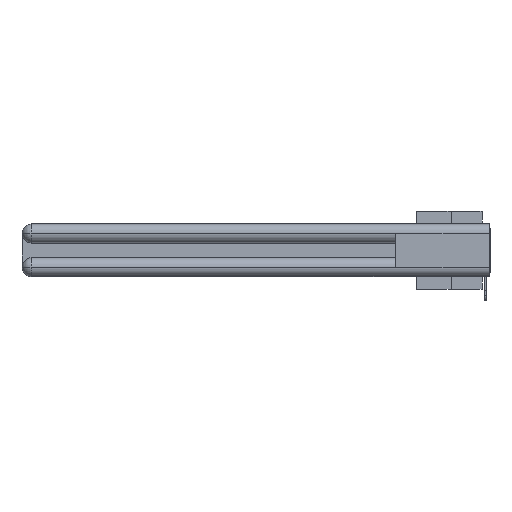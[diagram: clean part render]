
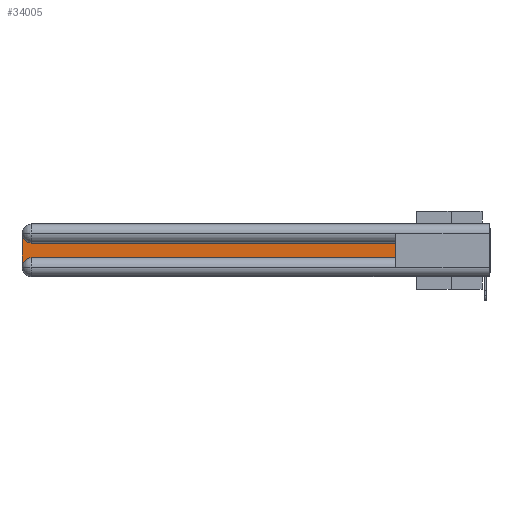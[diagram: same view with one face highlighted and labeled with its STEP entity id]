
A CAD part, left-side view. The second image highlights one B-rep face of the part: STEP entity #34005.
In plain terms, the highlighted planar face has unit normal (-1, 0, 0).
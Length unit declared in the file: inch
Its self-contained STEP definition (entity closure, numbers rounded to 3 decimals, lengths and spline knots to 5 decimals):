
#265 = DIRECTION ( 'NONE',  ( 1., 0., 0. ) ) ;
#384 = CARTESIAN_POINT ( 'NONE',  ( 0.075, 2.94, -0.2775 ) ) ;
#1418 = DIRECTION ( 'NONE',  ( 0., 0., 1. ) ) ;
#1859 = FACE_OUTER_BOUND ( 'NONE', #2344, .T. ) ;
#2344 = EDGE_LOOP ( 'NONE', ( #36586, #9857, #8368, #4734, #7684, #28062 ) ) ;
#3530 = AXIS2_PLACEMENT_3D ( 'NONE', #37875, #265, #41005 ) ;
#4423 = AXIS2_PLACEMENT_3D ( 'NONE', #8294, #18045, #14731 ) ;
#4734 = ORIENTED_EDGE ( 'NONE', *, *, #36474, .T. ) ;
#7265 = DIRECTION ( 'NONE',  ( 1., 0., 0. ) ) ;
#7353 = VERTEX_POINT ( 'NONE', #28153 ) ;
#7684 = ORIENTED_EDGE ( 'NONE', *, *, #11044, .T. ) ;
#8294 = CARTESIAN_POINT ( 'NONE',  ( 0.075, 3., -0.1225 ) ) ;
#8368 = ORIENTED_EDGE ( 'NONE', *, *, #30786, .T. ) ;
#9474 = CARTESIAN_POINT ( 'NONE',  ( 0.075, 3., -0.2175 ) ) ;
#9786 = AXIS2_PLACEMENT_3D ( 'NONE', #384, #7265, #19921 ) ;
#9857 = ORIENTED_EDGE ( 'NONE', *, *, #31177, .T. ) ;
#10422 = LINE ( 'NONE', #29315, #27068 ) ;
#11022 = VERTEX_POINT ( 'NONE', #39094 ) ;
#11044 = EDGE_CURVE ( 'NONE', #16330, #7353, #10422, .T. ) ;
#12972 = DIRECTION ( 'NONE',  ( 0., 0., -1. ) ) ;
#13334 = DIRECTION ( 'NONE',  ( 0., -1., 0. ) ) ;
#14731 = DIRECTION ( 'NONE',  ( 0., 0., -1. ) ) ;
#15416 = CARTESIAN_POINT ( 'NONE',  ( 0.075, 0.6, -0.1225 ) ) ;
#15624 = CARTESIAN_POINT ( 'NONE',  ( 0.075, 2.94, -0.1225 ) ) ;
#16330 = VERTEX_POINT ( 'NONE', #22347 ) ;
#16804 = VECTOR ( 'NONE', #24823, 39.37008 ) ;
#18045 = DIRECTION ( 'NONE',  ( 1., 0., 0. ) ) ;
#19921 = DIRECTION ( 'NONE',  ( 0., 0., -1. ) ) ;
#21067 = VECTOR ( 'NONE', #1418, 39.37008 ) ;
#21129 = CARTESIAN_POINT ( 'NONE',  ( 0.075, 0.6, -0.2175 ) ) ;
#22330 = CARTESIAN_POINT ( 'NONE',  ( 0.075, 0.6, -0.1225 ) ) ;
#22347 = CARTESIAN_POINT ( 'NONE',  ( 0.075, 2.94, -0.2175 ) ) ;
#24222 = LINE ( 'NONE', #21129, #21067 ) ;
#24823 = DIRECTION ( 'NONE',  ( 0., 1., 0. ) ) ;
#27068 = VECTOR ( 'NONE', #13334, 39.37008 ) ;
#27660 = CIRCLE ( 'NONE', #9786, 0.06 ) ;
#28062 = ORIENTED_EDGE ( 'NONE', *, *, #36531, .T. ) ;
#28153 = CARTESIAN_POINT ( 'NONE',  ( 0.075, 0.6, -0.2175 ) ) ;
#28333 = VERTEX_POINT ( 'NONE', #39480 ) ;
#29315 = CARTESIAN_POINT ( 'NONE',  ( 0.075, 0.6, -0.2175 ) ) ;
#29894 = VERTEX_POINT ( 'NONE', #15624 ) ;
#30762 = EDGE_CURVE ( 'NONE', #38937, #29894, #34601, .T. ) ;
#30786 = EDGE_CURVE ( 'NONE', #28333, #11022, #31689, .T. ) ;
#31177 = EDGE_CURVE ( 'NONE', #29894, #28333, #39348, .T. ) ;
#31689 = LINE ( 'NONE', #9474, #32051 ) ;
#32051 = VECTOR ( 'NONE', #12972, 39.37008 ) ;
#34005 = ADVANCED_FACE ( 'NONE', ( #1859 ), #40291, .F. ) ;
#34601 = LINE ( 'NONE', #22330, #16804 ) ;
#36474 = EDGE_CURVE ( 'NONE', #11022, #16330, #27660, .T. ) ;
#36531 = EDGE_CURVE ( 'NONE', #7353, #38937, #24222, .T. ) ;
#36586 = ORIENTED_EDGE ( 'NONE', *, *, #30762, .T. ) ;
#37875 = CARTESIAN_POINT ( 'NONE',  ( 0.075, 2.94, -0.0625 ) ) ;
#38937 = VERTEX_POINT ( 'NONE', #15416 ) ;
#39094 = CARTESIAN_POINT ( 'NONE',  ( 0.075, 3., -0.2775 ) ) ;
#39348 = CIRCLE ( 'NONE', #3530, 0.06 ) ;
#39480 = CARTESIAN_POINT ( 'NONE',  ( 0.075, 3., -0.0625 ) ) ;
#40291 = PLANE ( 'NONE',  #4423 ) ;
#41005 = DIRECTION ( 'NONE',  ( 0., 0., -1. ) ) ;
